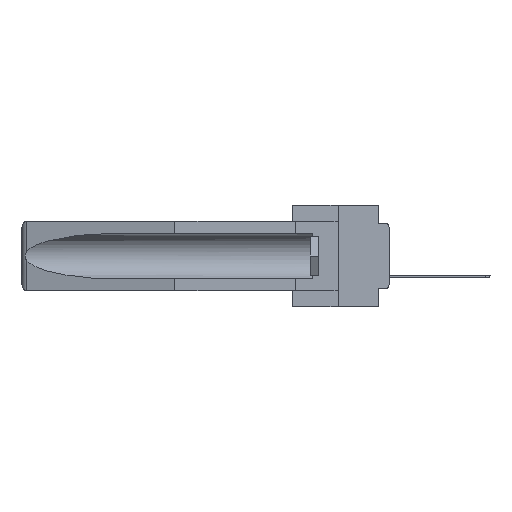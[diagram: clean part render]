
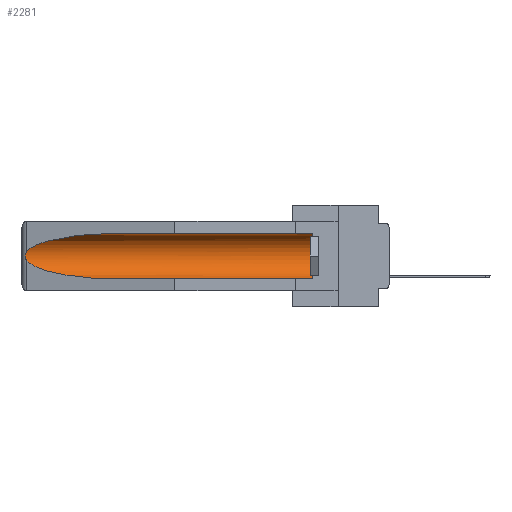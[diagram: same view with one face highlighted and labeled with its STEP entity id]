
A CAD part, left-side view. The second image highlights one B-rep face of the part: STEP entity #2281.
In plain terms, the highlighted cylindrical face has radius 2.857 mm (diameter 5.715 mm), a partial arc.
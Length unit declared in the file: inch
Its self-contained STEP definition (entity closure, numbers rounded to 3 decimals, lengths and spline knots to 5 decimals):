
#597 = ORIENTED_EDGE ( 'NONE', *, *, #28080, .T. ) ;
#680 = FACE_OUTER_BOUND ( 'NONE', #30578, .T. ) ;
#842 = VERTEX_POINT ( 'NONE', #35080 ) ;
#1123 = CARTESIAN_POINT ( 'NONE',  ( 0.26537, 1.52718, -0.14972 ) ) ;
#1248 = CARTESIAN_POINT ( 'NONE',  ( 0.2675, 1.53308, -0.16763 ) ) ;
#1457 = CARTESIAN_POINT ( 'NONE',  ( 0.26537, 1.52718, -0.19328 ) ) ;
#2218 = EDGE_CURVE ( 'NONE', #12311, #13312, #11089, .T. ) ;
#2281 = ADVANCED_FACE ( 'NONE', ( #680 ), #18543, .F. ) ;
#2363 = CARTESIAN_POINT ( 'NONE',  ( 0.155, 0.126, -0.284 ) ) ;
#2520 = ORIENTED_EDGE ( 'NONE', *, *, #10776, .T. ) ;
#2792 = CARTESIAN_POINT ( 'NONE',  ( 0.26537, 1.52718, -0.19328 ) ) ;
#3042 = LINE ( 'NONE', #7300, #15940 ) ;
#5872 = CARTESIAN_POINT ( 'NONE',  ( 0.26537, 1.52718, -0.14972 ) ) ;
#6114 = AXIS2_PLACEMENT_3D ( 'NONE', #25203, #8048, #28071 ) ;
#6135 = CARTESIAN_POINT ( 'NONE',  ( 0.155, 1.07973, -0.284 ) ) ;
#6721 =( BOUNDED_CURVE ( )  B_SPLINE_CURVE ( 3, ( #13641, #13257, #33663, #7793 ),
 .UNSPECIFIED., .F., .F. ) 
 B_SPLINE_CURVE_WITH_KNOTS ( ( 4, 4 ),
 ( 4.71239, 6.08839 ),
 .UNSPECIFIED. ) 
 CURVE ( )  GEOMETRIC_REPRESENTATION_ITEM ( )  RATIONAL_B_SPLINE_CURVE ( ( 1., 0.848, 0.848, 1. ) ) 
 REPRESENTATION_ITEM ( '' )  );
#7300 = CARTESIAN_POINT ( 'NONE',  ( 0.155, -0.30754, -0.059 ) ) ;
#7793 = CARTESIAN_POINT ( 'NONE',  ( 0.26537, 1.52718, -0.14972 ) ) ;
#8048 = DIRECTION ( 'NONE',  ( 0., -1., 0. ) ) ;
#10776 = EDGE_CURVE ( 'NONE', #22510, #842, #3042, .T. ) ;
#11089 = B_SPLINE_CURVE_WITH_KNOTS ( 'NONE', 3,
 ( #1123, #29557, #35160, #29433, #1248, #18040, #32796, #35695, #21073, #23953 ),
 .UNSPECIFIED., .F., .F.,
 ( 4, 2, 2, 2, 4 ),
 ( 0., 0.00029, 0.00058, 0.00087, 0.00117 ),
 .UNSPECIFIED. ) ;
#11626 = DIRECTION ( 'NONE',  ( 0., 1., 0. ) ) ;
#12044 = CARTESIAN_POINT ( 'NONE',  ( 0.155, 0.126, -0.059 ) ) ;
#12311 = VERTEX_POINT ( 'NONE', #5872 ) ;
#13257 = CARTESIAN_POINT ( 'NONE',  ( 0.21114, 1.30732, -0.059 ) ) ;
#13312 = VERTEX_POINT ( 'NONE', #1457 ) ;
#13641 = CARTESIAN_POINT ( 'NONE',  ( 0.155, 1.07973, -0.059 ) ) ;
#14166 = CARTESIAN_POINT ( 'NONE',  ( 0.25451, 1.48313, -0.24835 ) ) ;
#14510 = CARTESIAN_POINT ( 'NONE',  ( 0.155, 1.07973, -0.284 ) ) ;
#15933 = DIRECTION ( 'NONE',  ( 0., 1., 0. ) ) ;
#15940 = VECTOR ( 'NONE', #11626, 39.37008 ) ;
#16515 = AXIS2_PLACEMENT_3D ( 'NONE', #33190, #15933, #21957 ) ;
#18040 = CARTESIAN_POINT ( 'NONE',  ( 0.2675, 1.53308, -0.17534 ) ) ;
#18205 = VERTEX_POINT ( 'NONE', #2363 ) ;
#18312 = EDGE_CURVE ( 'NONE', #18205, #22510, #23290, .T. ) ;
#18543 = CYLINDRICAL_SURFACE ( 'NONE', #16515, 0.1125 ) ;
#21073 = CARTESIAN_POINT ( 'NONE',  ( 0.26597, 1.5296, -0.19026 ) ) ;
#21513 = ORIENTED_EDGE ( 'NONE', *, *, #18312, .T. ) ;
#21957 = DIRECTION ( 'NONE',  ( 0., 0., 1. ) ) ;
#22510 = VERTEX_POINT ( 'NONE', #12044 ) ;
#23290 = CIRCLE ( 'NONE', #6114, 0.1125 ) ;
#23395 = CARTESIAN_POINT ( 'NONE',  ( 0.21114, 1.30732, -0.284 ) ) ;
#23953 = CARTESIAN_POINT ( 'NONE',  ( 0.26537, 1.52718, -0.19328 ) ) ;
#25203 = CARTESIAN_POINT ( 'NONE',  ( 0.155, 0.126, -0.1715 ) ) ;
#26423 = VERTEX_POINT ( 'NONE', #6135 ) ;
#27636 = EDGE_CURVE ( 'NONE', #13312, #26423, #32124, .T. ) ;
#27976 = ORIENTED_EDGE ( 'NONE', *, *, #31704, .F. ) ;
#28071 = DIRECTION ( 'NONE',  ( 0., 0., 1. ) ) ;
#28080 = EDGE_CURVE ( 'NONE', #842, #12311, #6721, .T. ) ;
#29282 = CARTESIAN_POINT ( 'NONE',  ( 0.155, -0.30754, -0.284 ) ) ;
#29433 = CARTESIAN_POINT ( 'NONE',  ( 0.2673, 1.5327, -0.16383 ) ) ;
#29557 = CARTESIAN_POINT ( 'NONE',  ( 0.26597, 1.52961, -0.15275 ) ) ;
#30578 = EDGE_LOOP ( 'NONE', ( #597, #34935, #34322, #27976, #21513, #2520 ) ) ;
#31169 = VECTOR ( 'NONE', #35672, 39.37008 ) ;
#31704 = EDGE_CURVE ( 'NONE', #18205, #26423, #32454, .T. ) ;
#32124 =( BOUNDED_CURVE ( )  B_SPLINE_CURVE ( 3, ( #2792, #14166, #23395, #14510 ),
 .UNSPECIFIED., .F., .F. ) 
 B_SPLINE_CURVE_WITH_KNOTS ( ( 4, 4 ),
 ( 0.1948, 1.5708 ),
 .UNSPECIFIED. ) 
 CURVE ( )  GEOMETRIC_REPRESENTATION_ITEM ( )  RATIONAL_B_SPLINE_CURVE ( ( 1., 0.848, 0.848, 1. ) ) 
 REPRESENTATION_ITEM ( '' )  );
#32454 = LINE ( 'NONE', #29282, #31169 ) ;
#32796 = CARTESIAN_POINT ( 'NONE',  ( 0.2673, 1.53269, -0.17917 ) ) ;
#33190 = CARTESIAN_POINT ( 'NONE',  ( 0.155, -0.30754, -0.1715 ) ) ;
#33663 = CARTESIAN_POINT ( 'NONE',  ( 0.25451, 1.48313, -0.09465 ) ) ;
#34322 = ORIENTED_EDGE ( 'NONE', *, *, #27636, .T. ) ;
#34935 = ORIENTED_EDGE ( 'NONE', *, *, #2218, .T. ) ;
#35080 = CARTESIAN_POINT ( 'NONE',  ( 0.155, 1.07973, -0.059 ) ) ;
#35160 = CARTESIAN_POINT ( 'NONE',  ( 0.26654, 1.53092, -0.15636 ) ) ;
#35672 = DIRECTION ( 'NONE',  ( 0., 1., 0. ) ) ;
#35695 = CARTESIAN_POINT ( 'NONE',  ( 0.26655, 1.53094, -0.18657 ) ) ;
